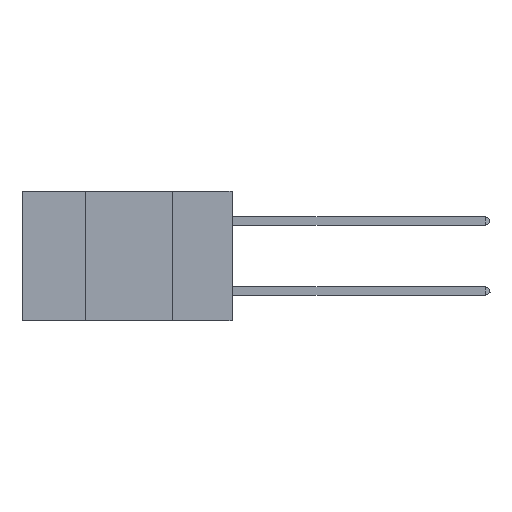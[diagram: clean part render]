
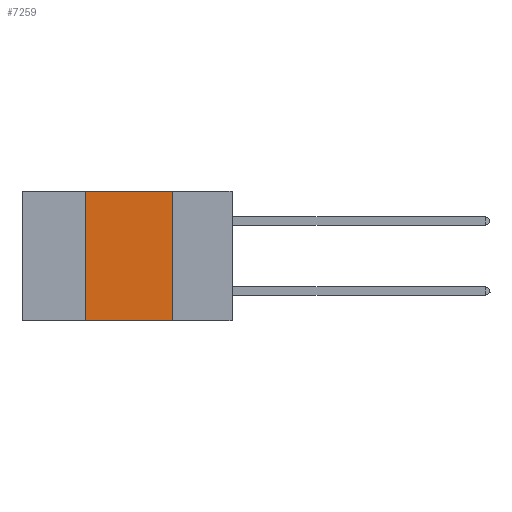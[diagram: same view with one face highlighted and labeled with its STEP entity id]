
A CAD part, left-side view. The second image highlights one B-rep face of the part: STEP entity #7259.
In plain terms, the highlighted planar face has unit normal (-1, 0, 0).
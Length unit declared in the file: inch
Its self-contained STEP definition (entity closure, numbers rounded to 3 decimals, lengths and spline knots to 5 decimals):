
#560 = EDGE_CURVE ( 'NONE', #4781, #15176, #7824, .T. ) ;
#1045 = EDGE_CURVE ( 'NONE', #5836, #9273, #11424, .T. ) ;
#1443 = DIRECTION ( 'NONE',  ( 0., -1., 0. ) ) ;
#2910 = VECTOR ( 'NONE', #15752, 39.37008 ) ;
#3042 = DIRECTION ( 'NONE',  ( 0., 0., -1. ) ) ;
#3432 = CARTESIAN_POINT ( 'NONE',  ( 0., 0.42, -0.37 ) ) ;
#3552 = VECTOR ( 'NONE', #1443, 39.37008 ) ;
#4623 = CARTESIAN_POINT ( 'NONE',  ( 0., 0.6, 0. ) ) ;
#4781 = VERTEX_POINT ( 'NONE', #3432 ) ;
#5808 = CARTESIAN_POINT ( 'NONE',  ( 0., 0.42, 0. ) ) ;
#5836 = VERTEX_POINT ( 'NONE', #5808 ) ;
#6604 = VECTOR ( 'NONE', #8448, 39.37008 ) ;
#6647 = CARTESIAN_POINT ( 'NONE',  ( 0., 0.6, -0.37 ) ) ;
#7219 = VECTOR ( 'NONE', #3042, 39.37008 ) ;
#7243 = DIRECTION ( 'NONE',  ( 1., 0., 0. ) ) ;
#7259 = ADVANCED_FACE ( 'NONE', ( #8473 ), #16005, .F. ) ;
#7634 = LINE ( 'NONE', #12090, #7219 ) ;
#7815 = EDGE_CURVE ( 'NONE', #4781, #5836, #10060, .T. ) ;
#7824 = LINE ( 'NONE', #6647, #3552 ) ;
#8100 = ORIENTED_EDGE ( 'NONE', *, *, #14539, .F. ) ;
#8448 = DIRECTION ( 'NONE',  ( 0., 0., 1. ) ) ;
#8473 = FACE_OUTER_BOUND ( 'NONE', #8859, .T. ) ;
#8859 = EDGE_LOOP ( 'NONE', ( #8100, #13728, #14087, #12788 ) ) ;
#9273 = VERTEX_POINT ( 'NONE', #10615 ) ;
#10060 = LINE ( 'NONE', #16195, #6604 ) ;
#10615 = CARTESIAN_POINT ( 'NONE',  ( 0., 0.17, 0. ) ) ;
#11424 = LINE ( 'NONE', #14511, #2910 ) ;
#12090 = CARTESIAN_POINT ( 'NONE',  ( 0., 0.17, 0. ) ) ;
#12238 = CARTESIAN_POINT ( 'NONE',  ( 0., 0.17, -0.37 ) ) ;
#12507 = AXIS2_PLACEMENT_3D ( 'NONE', #4623, #7243, #16286 ) ;
#12788 = ORIENTED_EDGE ( 'NONE', *, *, #560, .T. ) ;
#13728 = ORIENTED_EDGE ( 'NONE', *, *, #1045, .F. ) ;
#14087 = ORIENTED_EDGE ( 'NONE', *, *, #7815, .F. ) ;
#14511 = CARTESIAN_POINT ( 'NONE',  ( 0., 0.6, 0. ) ) ;
#14539 = EDGE_CURVE ( 'NONE', #9273, #15176, #7634, .T. ) ;
#15176 = VERTEX_POINT ( 'NONE', #12238 ) ;
#15752 = DIRECTION ( 'NONE',  ( 0., -1., 0. ) ) ;
#16005 = PLANE ( 'NONE',  #12507 ) ;
#16195 = CARTESIAN_POINT ( 'NONE',  ( 0., 0.42, 0. ) ) ;
#16286 = DIRECTION ( 'NONE',  ( 0., 0., -1. ) ) ;
